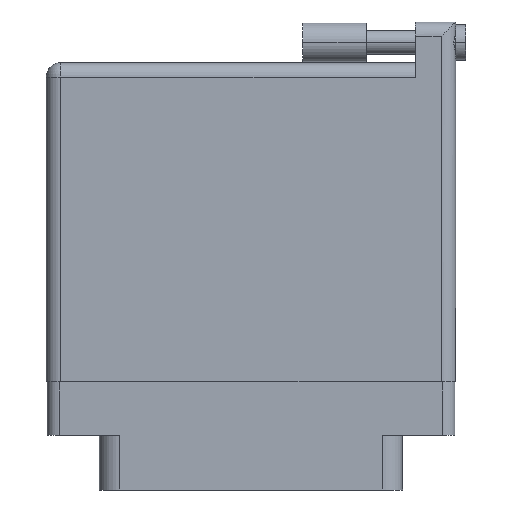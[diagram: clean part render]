
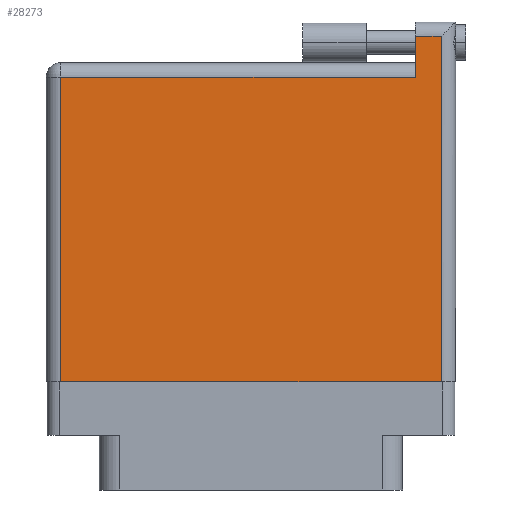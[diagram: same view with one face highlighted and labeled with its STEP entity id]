
A CAD part, front view. The second image highlights one B-rep face of the part: STEP entity #28273.
In plain terms, the highlighted face is planar.
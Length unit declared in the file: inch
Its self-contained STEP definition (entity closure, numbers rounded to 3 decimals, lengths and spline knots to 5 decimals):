
#187 = CARTESIAN_POINT ( 'NONE',  ( 1.811, 1.496, 0. ) ) ;
#767 = CARTESIAN_POINT ( 'NONE',  ( 0., 1.696, 0. ) ) ;
#1018 = DIRECTION ( 'NONE',  ( -1., 0., 0. ) ) ;
#1853 = PLANE ( 'NONE',  #24996 ) ;
#1935 = LINE ( 'NONE', #19913, #7088 ) ;
#2109 = DIRECTION ( 'NONE',  ( 0., 1., 0. ) ) ;
#4797 = EDGE_CURVE ( 'NONE', #17057, #18475, #26905, .T. ) ;
#5412 = VECTOR ( 'NONE', #22360, 39.37008 ) ;
#6113 = DIRECTION ( 'NONE',  ( 0., -1., 0. ) ) ;
#6660 = ORIENTED_EDGE ( 'NONE', *, *, #4797, .T. ) ;
#6807 = EDGE_CURVE ( 'NONE', #18475, #23121, #1935, .T. ) ;
#7088 = VECTOR ( 'NONE', #2109, 39.37008 ) ;
#9955 = DIRECTION ( 'NONE',  ( 1., 0., 0. ) ) ;
#10479 = VERTEX_POINT ( 'NONE', #187 ) ;
#11006 = DIRECTION ( 'NONE',  ( -1., 0., 0. ) ) ;
#11278 = FACE_OUTER_BOUND ( 'NONE', #36480, .T. ) ;
#11321 = ORIENTED_EDGE ( 'NONE', *, *, #14595, .T. ) ;
#12118 = VERTEX_POINT ( 'NONE', #29658 ) ;
#13826 = CARTESIAN_POINT ( 'NONE',  ( 1.938, 0., 0. ) ) ;
#13886 = LINE ( 'NONE', #14514, #35915 ) ;
#14514 = CARTESIAN_POINT ( 'NONE',  ( 0., 1.496, 0. ) ) ;
#14595 = EDGE_CURVE ( 'NONE', #12118, #10479, #32570, .T. ) ;
#16501 = CARTESIAN_POINT ( 'NONE',  ( 1.811, 1.766, 0. ) ) ;
#16750 = ORIENTED_EDGE ( 'NONE', *, *, #31940, .T. ) ;
#17057 = VERTEX_POINT ( 'NONE', #21334 ) ;
#18263 = ORIENTED_EDGE ( 'NONE', *, *, #22293, .T. ) ;
#18475 = VERTEX_POINT ( 'NONE', #13826 ) ;
#19913 = CARTESIAN_POINT ( 'NONE',  ( 1.938, 1.766, 0. ) ) ;
#20903 = CARTESIAN_POINT ( 'NONE',  ( 0.07, 0., 0. ) ) ;
#21334 = CARTESIAN_POINT ( 'NONE',  ( 0.07, 0., 0. ) ) ;
#22239 = VECTOR ( 'NONE', #9955, 39.37008 ) ;
#22293 = EDGE_CURVE ( 'NONE', #27715, #17057, #25841, .T. ) ;
#22360 = DIRECTION ( 'NONE',  ( 0., -1., 0. ) ) ;
#22414 = CARTESIAN_POINT ( 'NONE',  ( 1.938, 1.696, 0. ) ) ;
#22936 = EDGE_CURVE ( 'NONE', #23121, #12118, #28169, .T. ) ;
#23121 = VERTEX_POINT ( 'NONE', #22414 ) ;
#23603 = CARTESIAN_POINT ( 'NONE',  ( 0.07, 1.496, 0. ) ) ;
#24915 = ORIENTED_EDGE ( 'NONE', *, *, #22936, .T. ) ;
#24996 = AXIS2_PLACEMENT_3D ( 'NONE', #34706, #32075, #11006 ) ;
#25739 = DIRECTION ( 'NONE',  ( -1., 0., 0. ) ) ;
#25841 = LINE ( 'NONE', #20903, #28203 ) ;
#26453 = ORIENTED_EDGE ( 'NONE', *, *, #6807, .T. ) ;
#26905 = LINE ( 'NONE', #33251, #22239 ) ;
#27715 = VERTEX_POINT ( 'NONE', #23603 ) ;
#28169 = LINE ( 'NONE', #767, #30480 ) ;
#28203 = VECTOR ( 'NONE', #6113, 39.37008 ) ;
#28273 = ADVANCED_FACE ( 'NONE', ( #11278 ), #1853, .F. ) ;
#29658 = CARTESIAN_POINT ( 'NONE',  ( 1.811, 1.696, 0. ) ) ;
#30480 = VECTOR ( 'NONE', #1018, 39.37008 ) ;
#31940 = EDGE_CURVE ( 'NONE', #10479, #27715, #13886, .T. ) ;
#32075 = DIRECTION ( 'NONE',  ( 0., 0., -1. ) ) ;
#32570 = LINE ( 'NONE', #16501, #5412 ) ;
#33251 = CARTESIAN_POINT ( 'NONE',  ( 0., 0., 0. ) ) ;
#34706 = CARTESIAN_POINT ( 'NONE',  ( 0., 1.566, 0. ) ) ;
#35915 = VECTOR ( 'NONE', #25739, 39.37008 ) ;
#36480 = EDGE_LOOP ( 'NONE', ( #6660, #26453, #24915, #11321, #16750, #18263 ) ) ;
